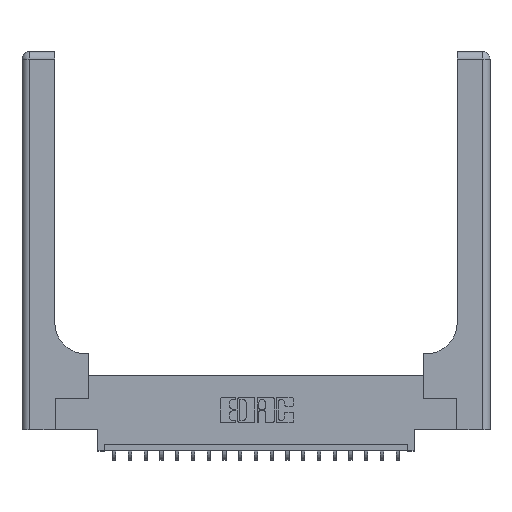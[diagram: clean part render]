
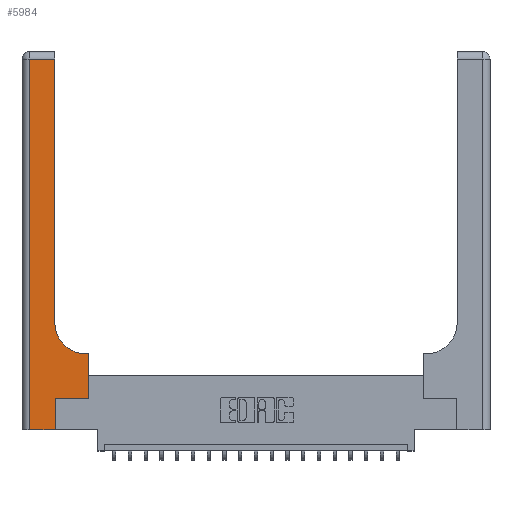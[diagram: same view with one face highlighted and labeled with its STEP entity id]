
A CAD part, top view. The second image highlights one B-rep face of the part: STEP entity #5984.
In plain terms, the highlighted planar face has unit normal (0, 0, 1).
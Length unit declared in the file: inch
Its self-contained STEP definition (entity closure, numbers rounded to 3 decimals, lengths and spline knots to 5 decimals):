
#114 = VECTOR ( 'NONE', #8156, 39.37008 ) ;
#131 = ORIENTED_EDGE ( 'NONE', *, *, #11711, .T. ) ;
#657 = LINE ( 'NONE', #16897, #1797 ) ;
#909 = CARTESIAN_POINT ( 'NONE',  ( 0.26, 3., 0.37 ) ) ;
#994 = VERTEX_POINT ( 'NONE', #8806 ) ;
#1221 = EDGE_CURVE ( 'NONE', #994, #15839, #2357, .T. ) ;
#1797 = VECTOR ( 'NONE', #6854, 39.37008 ) ;
#2315 = ORIENTED_EDGE ( 'NONE', *, *, #4568, .T. ) ;
#2357 = LINE ( 'NONE', #909, #11664 ) ;
#2468 = LINE ( 'NONE', #7293, #4295 ) ;
#2647 = VECTOR ( 'NONE', #3355, 39.37008 ) ;
#2709 = DIRECTION ( 'NONE',  ( 1., 0., 0. ) ) ;
#2730 = CARTESIAN_POINT ( 'NONE',  ( 0.265, 0., 0.37 ) ) ;
#3334 = LINE ( 'NONE', #9406, #11893 ) ;
#3355 = DIRECTION ( 'NONE',  ( -1., 0., 0. ) ) ;
#4194 = VERTEX_POINT ( 'NONE', #7368 ) ;
#4295 = VECTOR ( 'NONE', #10432, 39.37008 ) ;
#4568 = EDGE_CURVE ( 'NONE', #15839, #16000, #17728, .T. ) ;
#4812 = CIRCLE ( 'NONE', #7750, 0.25 ) ;
#4897 = CARTESIAN_POINT ( 'NONE',  ( 0.06, 2.94, 0.37 ) ) ;
#5341 = EDGE_CURVE ( 'NONE', #16000, #19389, #2468, .T. ) ;
#5556 = CARTESIAN_POINT ( 'NONE',  ( 0., 3., 0.37 ) ) ;
#5592 = CARTESIAN_POINT ( 'NONE',  ( 0.51, 0.6, 0.37 ) ) ;
#5984 = ADVANCED_FACE ( 'NONE', ( #13507 ), #19916, .F. ) ;
#6204 = CARTESIAN_POINT ( 'NONE',  ( 0., 2.94, 0.37 ) ) ;
#6542 = CARTESIAN_POINT ( 'NONE',  ( 0.528, 0.25, 0.37 ) ) ;
#6688 = CARTESIAN_POINT ( 'NONE',  ( 0., 0., 0.37 ) ) ;
#6854 = DIRECTION ( 'NONE',  ( 1., 0., 0. ) ) ;
#7293 = CARTESIAN_POINT ( 'NONE',  ( 0.06, 3., 0.37 ) ) ;
#7368 = CARTESIAN_POINT ( 'NONE',  ( 0.265, 0., 0.37 ) ) ;
#7462 = ORIENTED_EDGE ( 'NONE', *, *, #5341, .T. ) ;
#7750 = AXIS2_PLACEMENT_3D ( 'NONE', #20129, #15180, #2709 ) ;
#7762 = DIRECTION ( 'NONE',  ( 0., 1., 0. ) ) ;
#7795 = ORIENTED_EDGE ( 'NONE', *, *, #15116, .T. ) ;
#8042 = LINE ( 'NONE', #6688, #114 ) ;
#8156 = DIRECTION ( 'NONE',  ( 1., 0., 0. ) ) ;
#8806 = CARTESIAN_POINT ( 'NONE',  ( 0.26, 0.85, 0.37 ) ) ;
#9406 = CARTESIAN_POINT ( 'NONE',  ( 0.26, 0.6, 0.37 ) ) ;
#9957 = DIRECTION ( 'NONE',  ( 0., 0., -1. ) ) ;
#10018 = VERTEX_POINT ( 'NONE', #6542 ) ;
#10432 = DIRECTION ( 'NONE',  ( 0., -1., 0. ) ) ;
#10635 = CARTESIAN_POINT ( 'NONE',  ( 0.06, 0., 0.37 ) ) ;
#10797 = EDGE_CURVE ( 'NONE', #19389, #4194, #8042, .T. ) ;
#11106 = ORIENTED_EDGE ( 'NONE', *, *, #15548, .T. ) ;
#11664 = VECTOR ( 'NONE', #16627, 39.37008 ) ;
#11711 = EDGE_CURVE ( 'NONE', #13100, #994, #4812, .T. ) ;
#11893 = VECTOR ( 'NONE', #20538, 39.37008 ) ;
#11945 = DIRECTION ( 'NONE',  ( -1., 0., 0. ) ) ;
#12599 = ORIENTED_EDGE ( 'NONE', *, *, #17863, .T. ) ;
#13026 = EDGE_CURVE ( 'NONE', #16157, #10018, #657, .T. ) ;
#13100 = VERTEX_POINT ( 'NONE', #5592 ) ;
#13507 = FACE_OUTER_BOUND ( 'NONE', #16552, .T. ) ;
#13958 = CARTESIAN_POINT ( 'NONE',  ( 0.528, 0.25, 0.37 ) ) ;
#15116 = EDGE_CURVE ( 'NONE', #4194, #16157, #15616, .T. ) ;
#15180 = DIRECTION ( 'NONE',  ( 0., 0., -1. ) ) ;
#15345 = ORIENTED_EDGE ( 'NONE', *, *, #1221, .T. ) ;
#15548 = EDGE_CURVE ( 'NONE', #20373, #13100, #3334, .T. ) ;
#15616 = LINE ( 'NONE', #2730, #18940 ) ;
#15716 = DIRECTION ( 'NONE',  ( 0., 1., 0. ) ) ;
#15839 = VERTEX_POINT ( 'NONE', #20408 ) ;
#16000 = VERTEX_POINT ( 'NONE', #4897 ) ;
#16157 = VERTEX_POINT ( 'NONE', #19558 ) ;
#16552 = EDGE_LOOP ( 'NONE', ( #15345, #2315, #7462, #18929, #7795, #19296, #12599, #11106, #131 ) ) ;
#16627 = DIRECTION ( 'NONE',  ( 0., 1., 0. ) ) ;
#16897 = CARTESIAN_POINT ( 'NONE',  ( 0.265, 0.25, 0.37 ) ) ;
#17198 = LINE ( 'NONE', #13958, #20046 ) ;
#17728 = LINE ( 'NONE', #6204, #2647 ) ;
#17863 = EDGE_CURVE ( 'NONE', #10018, #20373, #17198, .T. ) ;
#17899 = CARTESIAN_POINT ( 'NONE',  ( 0.528, 0.6, 0.37 ) ) ;
#18929 = ORIENTED_EDGE ( 'NONE', *, *, #10797, .T. ) ;
#18940 = VECTOR ( 'NONE', #15716, 39.37008 ) ;
#19296 = ORIENTED_EDGE ( 'NONE', *, *, #13026, .T. ) ;
#19389 = VERTEX_POINT ( 'NONE', #10635 ) ;
#19558 = CARTESIAN_POINT ( 'NONE',  ( 0.265, 0.25, 0.37 ) ) ;
#19916 = PLANE ( 'NONE',  #20061 ) ;
#20046 = VECTOR ( 'NONE', #7762, 39.37008 ) ;
#20061 = AXIS2_PLACEMENT_3D ( 'NONE', #5556, #9957, #11945 ) ;
#20129 = CARTESIAN_POINT ( 'NONE',  ( 0.51, 0.85, 0.37 ) ) ;
#20373 = VERTEX_POINT ( 'NONE', #17899 ) ;
#20408 = CARTESIAN_POINT ( 'NONE',  ( 0.26, 2.94, 0.37 ) ) ;
#20538 = DIRECTION ( 'NONE',  ( -1., 0., 0. ) ) ;
